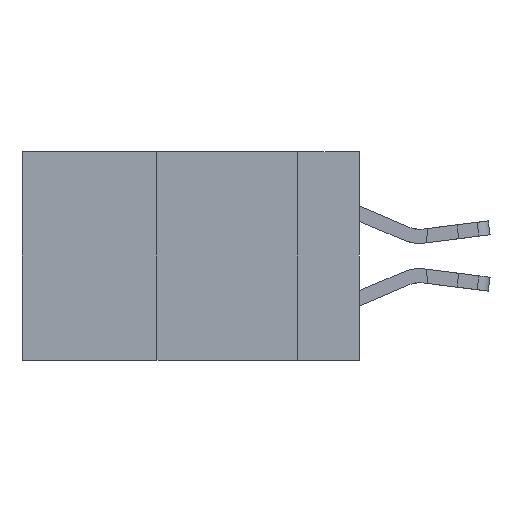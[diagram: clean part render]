
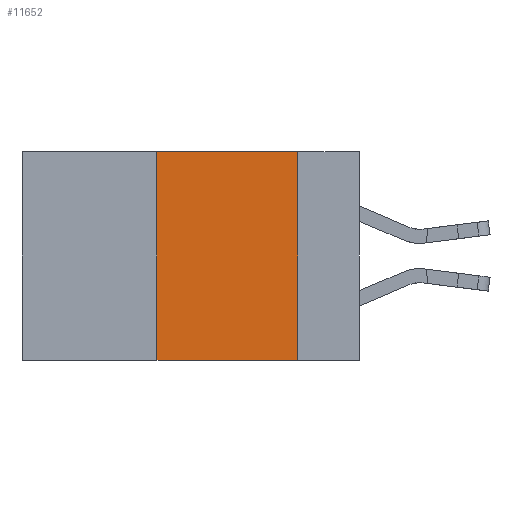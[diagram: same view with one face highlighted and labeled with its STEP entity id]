
A CAD part, left-side view. The second image highlights one B-rep face of the part: STEP entity #11652.
In plain terms, the highlighted planar face has unit normal (-1, 0, 0).
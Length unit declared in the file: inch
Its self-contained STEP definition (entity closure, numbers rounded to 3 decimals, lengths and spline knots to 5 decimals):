
#1456 = DIRECTION ( 'NONE',  ( 0., -1., 0. ) ) ;
#1698 = DIRECTION ( 'NONE',  ( 0., 0., 1. ) ) ;
#1991 = LINE ( 'NONE', #10050, #13701 ) ;
#2674 = CARTESIAN_POINT ( 'NONE',  ( 0., 0.36, -0.37 ) ) ;
#3606 = DIRECTION ( 'NONE',  ( 1., 0., 0. ) ) ;
#3913 = EDGE_CURVE ( 'NONE', #4886, #25231, #9700, .T. ) ;
#4886 = VERTEX_POINT ( 'NONE', #2674 ) ;
#5679 = DIRECTION ( 'NONE',  ( 0., 0., -1. ) ) ;
#5779 = CARTESIAN_POINT ( 'NONE',  ( 0., 0.36, 0. ) ) ;
#5988 = VECTOR ( 'NONE', #11157, 39.37008 ) ;
#6459 = ORIENTED_EDGE ( 'NONE', *, *, #15717, .F. ) ;
#9361 = AXIS2_PLACEMENT_3D ( 'NONE', #15427, #3606, #5679 ) ;
#9700 = LINE ( 'NONE', #13923, #14614 ) ;
#10050 = CARTESIAN_POINT ( 'NONE',  ( 0., 0.11, 0. ) ) ;
#10794 = CARTESIAN_POINT ( 'NONE',  ( 0., 0.6, 0. ) ) ;
#10953 = ORIENTED_EDGE ( 'NONE', *, *, #20105, .F. ) ;
#11157 = DIRECTION ( 'NONE',  ( 0., -1., 0. ) ) ;
#11652 = ADVANCED_FACE ( 'NONE', ( #25419 ), #26420, .F. ) ;
#12047 = CARTESIAN_POINT ( 'NONE',  ( 0., 0.11, -0.37 ) ) ;
#13350 = ORIENTED_EDGE ( 'NONE', *, *, #15339, .F. ) ;
#13701 = VECTOR ( 'NONE', #14198, 39.37008 ) ;
#13923 = CARTESIAN_POINT ( 'NONE',  ( 0., 0.6, -0.37 ) ) ;
#14198 = DIRECTION ( 'NONE',  ( 0., 0., -1. ) ) ;
#14614 = VECTOR ( 'NONE', #1456, 39.37008 ) ;
#14723 = VECTOR ( 'NONE', #1698, 39.37008 ) ;
#15078 = ORIENTED_EDGE ( 'NONE', *, *, #3913, .T. ) ;
#15339 = EDGE_CURVE ( 'NONE', #21820, #25231, #1991, .T. ) ;
#15427 = CARTESIAN_POINT ( 'NONE',  ( 0., 0.6, 0. ) ) ;
#15717 = EDGE_CURVE ( 'NONE', #4886, #25116, #16014, .T. ) ;
#16014 = LINE ( 'NONE', #5779, #14723 ) ;
#20105 = EDGE_CURVE ( 'NONE', #25116, #21820, #25503, .T. ) ;
#20900 = CARTESIAN_POINT ( 'NONE',  ( 0., 0.11, 0. ) ) ;
#21820 = VERTEX_POINT ( 'NONE', #20900 ) ;
#24355 = CARTESIAN_POINT ( 'NONE',  ( 0., 0.36, 0. ) ) ;
#25116 = VERTEX_POINT ( 'NONE', #24355 ) ;
#25231 = VERTEX_POINT ( 'NONE', #12047 ) ;
#25419 = FACE_OUTER_BOUND ( 'NONE', #26784, .T. ) ;
#25503 = LINE ( 'NONE', #10794, #5988 ) ;
#26420 = PLANE ( 'NONE',  #9361 ) ;
#26784 = EDGE_LOOP ( 'NONE', ( #13350, #10953, #6459, #15078 ) ) ;
